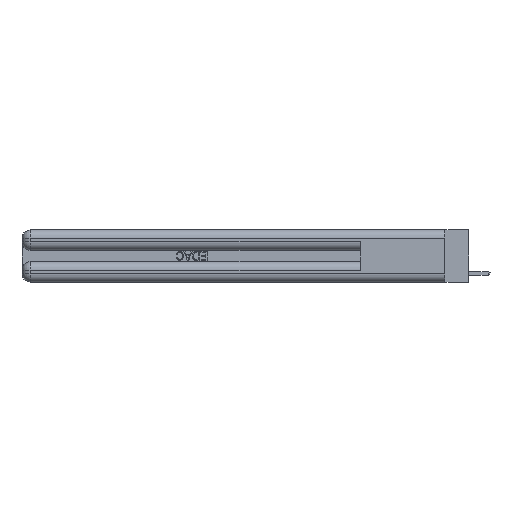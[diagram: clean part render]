
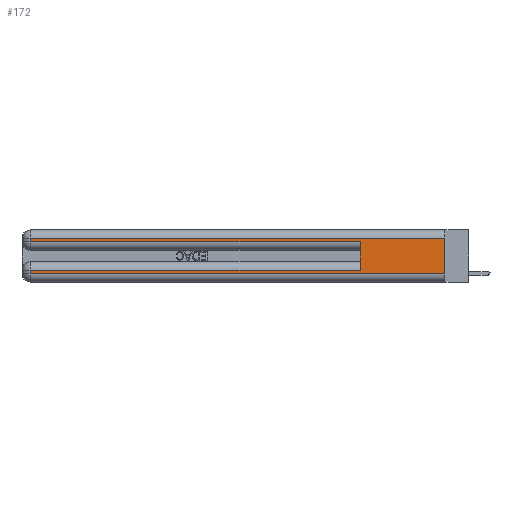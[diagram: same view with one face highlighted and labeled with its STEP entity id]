
A CAD part, left-side view. The second image highlights one B-rep face of the part: STEP entity #172.
In plain terms, the highlighted planar face has unit normal (-1, 0, 0).
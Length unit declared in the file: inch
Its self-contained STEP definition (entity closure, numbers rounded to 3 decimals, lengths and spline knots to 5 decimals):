
#172 = ADVANCED_FACE ( 'NONE', ( #24104 ), #724, .F. ) ;
#305 = CARTESIAN_POINT ( 'NONE',  ( 0., 0., 0.37 ) ) ;
#634 = CARTESIAN_POINT ( 'NONE',  ( 0., 0., 0.31 ) ) ;
#724 = PLANE ( 'NONE',  #29439 ) ;
#1320 = CARTESIAN_POINT ( 'NONE',  ( 0., 2.94, 0.06 ) ) ;
#1887 = CARTESIAN_POINT ( 'NONE',  ( 0., 2.94, 0.31 ) ) ;
#1911 = EDGE_CURVE ( 'NONE', #5499, #12944, #14278, .T. ) ;
#2006 = VERTEX_POINT ( 'NONE', #1887 ) ;
#3133 = VECTOR ( 'NONE', #7839, 39.37008 ) ;
#3738 = LINE ( 'NONE', #6476, #10711 ) ;
#3787 = LINE ( 'NONE', #9069, #26561 ) ;
#3788 = ORIENTED_EDGE ( 'NONE', *, *, #12017, .T. ) ;
#4633 = DIRECTION ( 'NONE',  ( 0., -1., 0. ) ) ;
#5499 = VERTEX_POINT ( 'NONE', #21837 ) ;
#6476 = CARTESIAN_POINT ( 'NONE',  ( 0., 0.6, 0.145 ) ) ;
#6690 = VECTOR ( 'NONE', #4633, 39.37008 ) ;
#7017 = VERTEX_POINT ( 'NONE', #634 ) ;
#7042 = DIRECTION ( 'NONE',  ( 0., 1., 0. ) ) ;
#7839 = DIRECTION ( 'NONE',  ( 0., 0., -1. ) ) ;
#8525 = DIRECTION ( 'NONE',  ( 0., 0., 1. ) ) ;
#8776 = DIRECTION ( 'NONE',  ( 0., 0., -1. ) ) ;
#9069 = CARTESIAN_POINT ( 'NONE',  ( 0., 0., 0.285 ) ) ;
#9337 = CARTESIAN_POINT ( 'NONE',  ( 0., 0., 0.085 ) ) ;
#9720 = CARTESIAN_POINT ( 'NONE',  ( 0., 0., 0.06 ) ) ;
#10711 = VECTOR ( 'NONE', #8525, 39.37008 ) ;
#11097 = DIRECTION ( 'NONE',  ( 1., 0., 0. ) ) ;
#11794 = CARTESIAN_POINT ( 'NONE',  ( 0., 2.94, 0.37 ) ) ;
#11908 = ORIENTED_EDGE ( 'NONE', *, *, #32810, .F. ) ;
#11919 = LINE ( 'NONE', #9720, #6690 ) ;
#12017 = EDGE_CURVE ( 'NONE', #2006, #33181, #20466, .T. ) ;
#12944 = VERTEX_POINT ( 'NONE', #26207 ) ;
#13055 = CARTESIAN_POINT ( 'NONE',  ( 0., 0.6, 0.285 ) ) ;
#13817 = DIRECTION ( 'NONE',  ( 0., 0., -1. ) ) ;
#14062 = VECTOR ( 'NONE', #31241, 39.37008 ) ;
#14122 = VERTEX_POINT ( 'NONE', #29294 ) ;
#14278 = LINE ( 'NONE', #9337, #27094 ) ;
#15273 = VERTEX_POINT ( 'NONE', #1320 ) ;
#15497 = ORIENTED_EDGE ( 'NONE', *, *, #29952, .F. ) ;
#15882 = CARTESIAN_POINT ( 'NONE',  ( 0., 0., 0.37 ) ) ;
#16353 = EDGE_CURVE ( 'NONE', #7017, #2006, #20002, .T. ) ;
#16961 = ORIENTED_EDGE ( 'NONE', *, *, #16353, .T. ) ;
#17289 = LINE ( 'NONE', #11794, #26887 ) ;
#19769 = ORIENTED_EDGE ( 'NONE', *, *, #21919, .T. ) ;
#20002 = LINE ( 'NONE', #30453, #21364 ) ;
#20466 = LINE ( 'NONE', #33502, #3133 ) ;
#20787 = LINE ( 'NONE', #305, #14062 ) ;
#21364 = VECTOR ( 'NONE', #7042, 39.37008 ) ;
#21729 = DIRECTION ( 'NONE',  ( 0., -1., 0. ) ) ;
#21837 = CARTESIAN_POINT ( 'NONE',  ( 0., 0.6, 0.085 ) ) ;
#21919 = EDGE_CURVE ( 'NONE', #33181, #31639, #3787, .T. ) ;
#23509 = ORIENTED_EDGE ( 'NONE', *, *, #28465, .T. ) ;
#23587 = EDGE_CURVE ( 'NONE', #12944, #15273, #17289, .T. ) ;
#24104 = FACE_OUTER_BOUND ( 'NONE', #25932, .T. ) ;
#25709 = CARTESIAN_POINT ( 'NONE',  ( 0., 2.94, 0.285 ) ) ;
#25932 = EDGE_LOOP ( 'NONE', ( #11908, #16961, #3788, #19769, #15497, #28246, #33671, #23509 ) ) ;
#26207 = CARTESIAN_POINT ( 'NONE',  ( 0., 2.94, 0.085 ) ) ;
#26561 = VECTOR ( 'NONE', #21729, 39.37008 ) ;
#26887 = VECTOR ( 'NONE', #8776, 39.37008 ) ;
#27094 = VECTOR ( 'NONE', #30210, 39.37008 ) ;
#28246 = ORIENTED_EDGE ( 'NONE', *, *, #1911, .T. ) ;
#28465 = EDGE_CURVE ( 'NONE', #15273, #14122, #11919, .T. ) ;
#29294 = CARTESIAN_POINT ( 'NONE',  ( 0., 0., 0.06 ) ) ;
#29439 = AXIS2_PLACEMENT_3D ( 'NONE', #15882, #11097, #13817 ) ;
#29952 = EDGE_CURVE ( 'NONE', #5499, #31639, #3738, .T. ) ;
#30210 = DIRECTION ( 'NONE',  ( 0., 1., 0. ) ) ;
#30453 = CARTESIAN_POINT ( 'NONE',  ( 0., 0., 0.31 ) ) ;
#31241 = DIRECTION ( 'NONE',  ( 0., 0., -1. ) ) ;
#31639 = VERTEX_POINT ( 'NONE', #13055 ) ;
#32810 = EDGE_CURVE ( 'NONE', #7017, #14122, #20787, .T. ) ;
#33181 = VERTEX_POINT ( 'NONE', #25709 ) ;
#33502 = CARTESIAN_POINT ( 'NONE',  ( 0., 2.94, 0.37 ) ) ;
#33671 = ORIENTED_EDGE ( 'NONE', *, *, #23587, .T. ) ;
